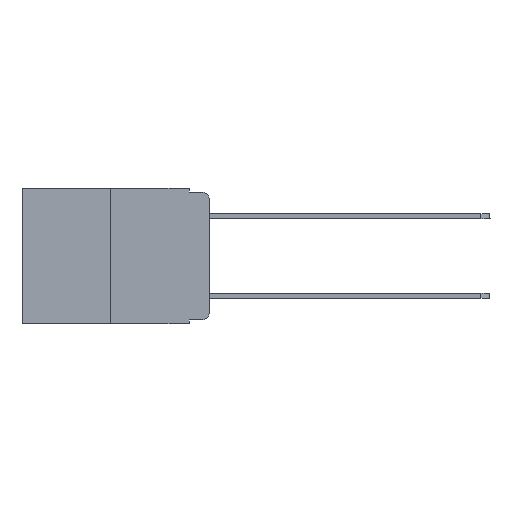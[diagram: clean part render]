
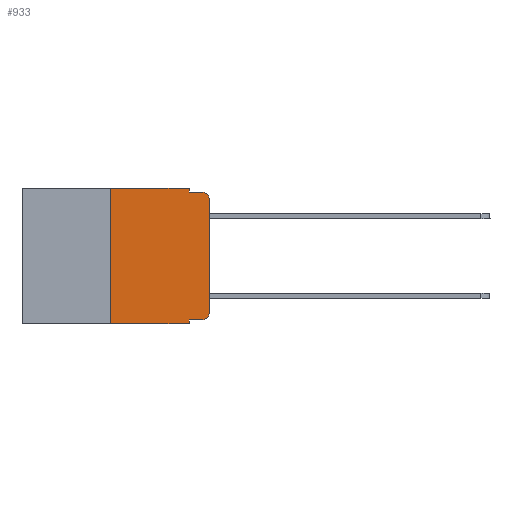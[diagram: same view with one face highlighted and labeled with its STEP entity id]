
A CAD part, left-side view. The second image highlights one B-rep face of the part: STEP entity #933.
In plain terms, the highlighted planar face has unit normal (-1, 0, 0).
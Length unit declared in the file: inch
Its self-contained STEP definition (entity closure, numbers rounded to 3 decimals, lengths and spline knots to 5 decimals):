
#302 = DIRECTION ( 'NONE',  ( 1., 0., 0. ) ) ;
#689 = DIRECTION ( 'NONE',  ( 0., 0., -1. ) ) ;
#933 = ADVANCED_FACE ( 'NONE', ( #17974 ), #2503, .F. ) ;
#1032 = VECTOR ( 'NONE', #15260, 39.37008 ) ;
#1218 = DIRECTION ( 'NONE',  ( 0., 0., -1. ) ) ;
#1393 = AXIS2_PLACEMENT_3D ( 'NONE', #12138, #302, #689 ) ;
#1690 = VERTEX_POINT ( 'NONE', #24012 ) ;
#2463 = DIRECTION ( 'NONE',  ( 0., 0., -1. ) ) ;
#2503 = PLANE ( 'NONE',  #1393 ) ;
#2758 = VECTOR ( 'NONE', #1218, 39.37008 ) ;
#2844 = ORIENTED_EDGE ( 'NONE', *, *, #18155, .T. ) ;
#2957 = VERTEX_POINT ( 'NONE', #14556 ) ;
#3079 = CARTESIAN_POINT ( 'NONE',  ( 0., 0.02, -0.313 ) ) ;
#3467 = DIRECTION ( 'NONE',  ( 0., 0., 1. ) ) ;
#3682 = ORIENTED_EDGE ( 'NONE', *, *, #21958, .T. ) ;
#3788 = EDGE_CURVE ( 'NONE', #14447, #2957, #8457, .T. ) ;
#3817 = CARTESIAN_POINT ( 'NONE',  ( 0., 0.051, -0.01 ) ) ;
#4000 = AXIS2_PLACEMENT_3D ( 'NONE', #3079, #18644, #20854 ) ;
#4094 = LINE ( 'NONE', #10237, #12550 ) ;
#4273 = CARTESIAN_POINT ( 'NONE',  ( 0., 0.02, -0.03 ) ) ;
#4788 = ORIENTED_EDGE ( 'NONE', *, *, #15605, .T. ) ;
#5105 = DIRECTION ( 'NONE',  ( 0., -1., 0. ) ) ;
#5526 = CARTESIAN_POINT ( 'NONE',  ( 0., 0.02, -0.333 ) ) ;
#6184 = VERTEX_POINT ( 'NONE', #20712 ) ;
#6798 = CARTESIAN_POINT ( 'NONE',  ( 0., 0.051, 0. ) ) ;
#7352 = VERTEX_POINT ( 'NONE', #24975 ) ;
#7567 = LINE ( 'NONE', #21099, #24034 ) ;
#7849 = EDGE_CURVE ( 'NONE', #6184, #12218, #13056, .T. ) ;
#8457 = LINE ( 'NONE', #6798, #1032 ) ;
#9156 = ORIENTED_EDGE ( 'NONE', *, *, #3788, .F. ) ;
#9498 = EDGE_CURVE ( 'NONE', #1690, #7352, #10308, .T. ) ;
#10237 = CARTESIAN_POINT ( 'NONE',  ( 0., 0.473, 0. ) ) ;
#10308 = LINE ( 'NONE', #13647, #24059 ) ;
#10971 = DIRECTION ( 'NONE',  ( 0., 0., 1. ) ) ;
#11133 = CARTESIAN_POINT ( 'NONE',  ( 0., 0.051, 0. ) ) ;
#12138 = CARTESIAN_POINT ( 'NONE',  ( 0., 0.473, 0. ) ) ;
#12168 = DIRECTION ( 'NONE',  ( 0., -1., 0. ) ) ;
#12218 = VERTEX_POINT ( 'NONE', #24885 ) ;
#12401 = ORIENTED_EDGE ( 'NONE', *, *, #16025, .T. ) ;
#12550 = VECTOR ( 'NONE', #12168, 39.37008 ) ;
#12729 = ORIENTED_EDGE ( 'NONE', *, *, #12746, .F. ) ;
#12746 = EDGE_CURVE ( 'NONE', #23617, #23839, #7567, .T. ) ;
#12864 = ORIENTED_EDGE ( 'NONE', *, *, #14626, .F. ) ;
#13056 = LINE ( 'NONE', #18884, #2758 ) ;
#13326 = VECTOR ( 'NONE', #23564, 39.37008 ) ;
#13647 = CARTESIAN_POINT ( 'NONE',  ( 0., 0., 0. ) ) ;
#13974 = CARTESIAN_POINT ( 'NONE',  ( 0., 0.051, -0.333 ) ) ;
#14039 = VERTEX_POINT ( 'NONE', #5526 ) ;
#14111 = EDGE_CURVE ( 'NONE', #23839, #14447, #4094, .T. ) ;
#14447 = VERTEX_POINT ( 'NONE', #11133 ) ;
#14556 = CARTESIAN_POINT ( 'NONE',  ( 0., 0.051, -0.01 ) ) ;
#14626 = EDGE_CURVE ( 'NONE', #2957, #17835, #21841, .T. ) ;
#15097 = CIRCLE ( 'NONE', #4000, 0.02 ) ;
#15260 = DIRECTION ( 'NONE',  ( 0., 0., -1. ) ) ;
#15605 = EDGE_CURVE ( 'NONE', #14039, #1690, #15097, .T. ) ;
#16025 = EDGE_CURVE ( 'NONE', #23617, #12218, #22760, .T. ) ;
#16170 = CARTESIAN_POINT ( 'NONE',  ( 0., 0.25, -0.343 ) ) ;
#17722 = VECTOR ( 'NONE', #5105, 39.37008 ) ;
#17835 = VERTEX_POINT ( 'NONE', #24674 ) ;
#17970 = DIRECTION ( 'NONE',  ( 0., -1., 0. ) ) ;
#17974 = FACE_OUTER_BOUND ( 'NONE', #22196, .T. ) ;
#18155 = EDGE_CURVE ( 'NONE', #7352, #17835, #20699, .T. ) ;
#18644 = DIRECTION ( 'NONE',  ( -1., 0., 0. ) ) ;
#18730 = ORIENTED_EDGE ( 'NONE', *, *, #9498, .T. ) ;
#18884 = CARTESIAN_POINT ( 'NONE',  ( 0., 0.051, 0. ) ) ;
#19430 = LINE ( 'NONE', #13974, #13326 ) ;
#20144 = ORIENTED_EDGE ( 'NONE', *, *, #14111, .F. ) ;
#20676 = AXIS2_PLACEMENT_3D ( 'NONE', #4273, #21673, #2463 ) ;
#20699 = CIRCLE ( 'NONE', #20676, 0.02 ) ;
#20712 = CARTESIAN_POINT ( 'NONE',  ( 0., 0.051, -0.333 ) ) ;
#20854 = DIRECTION ( 'NONE',  ( 0., 0., -1. ) ) ;
#21099 = CARTESIAN_POINT ( 'NONE',  ( 0., 0.25, 0. ) ) ;
#21673 = DIRECTION ( 'NONE',  ( -1., 0., 0. ) ) ;
#21841 = LINE ( 'NONE', #3817, #23312 ) ;
#21958 = EDGE_CURVE ( 'NONE', #6184, #14039, #19430, .T. ) ;
#22196 = EDGE_LOOP ( 'NONE', ( #18730, #2844, #12864, #9156, #20144, #12729, #12401, #22282, #3682, #4788 ) ) ;
#22282 = ORIENTED_EDGE ( 'NONE', *, *, #7849, .F. ) ;
#22760 = LINE ( 'NONE', #24560, #17722 ) ;
#23312 = VECTOR ( 'NONE', #17970, 39.37008 ) ;
#23564 = DIRECTION ( 'NONE',  ( 0., -1., 0. ) ) ;
#23617 = VERTEX_POINT ( 'NONE', #16170 ) ;
#23839 = VERTEX_POINT ( 'NONE', #24571 ) ;
#24012 = CARTESIAN_POINT ( 'NONE',  ( 0., 0., -0.313 ) ) ;
#24034 = VECTOR ( 'NONE', #3467, 39.37008 ) ;
#24059 = VECTOR ( 'NONE', #10971, 39.37008 ) ;
#24560 = CARTESIAN_POINT ( 'NONE',  ( 0., 0.473, -0.343 ) ) ;
#24571 = CARTESIAN_POINT ( 'NONE',  ( 0., 0.25, 0. ) ) ;
#24674 = CARTESIAN_POINT ( 'NONE',  ( 0., 0.02, -0.01 ) ) ;
#24885 = CARTESIAN_POINT ( 'NONE',  ( 0., 0.051, -0.343 ) ) ;
#24975 = CARTESIAN_POINT ( 'NONE',  ( 0., 0., -0.03 ) ) ;
